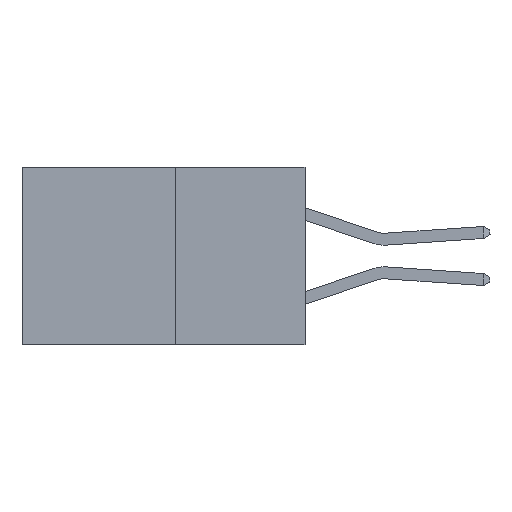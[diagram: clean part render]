
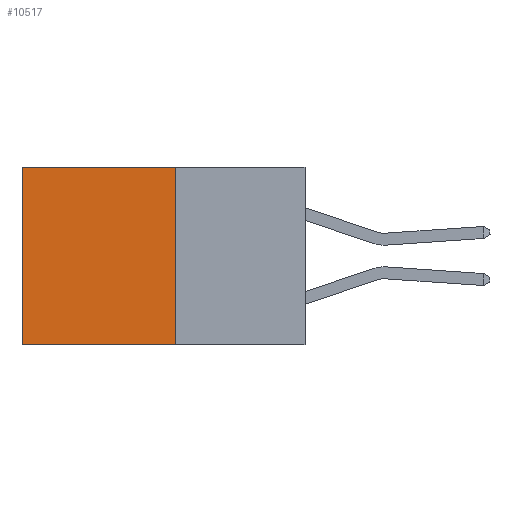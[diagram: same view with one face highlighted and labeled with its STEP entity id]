
A CAD part, left-side view. The second image highlights one B-rep face of the part: STEP entity #10517.
In plain terms, the highlighted planar face has unit normal (-1, 0, 0).
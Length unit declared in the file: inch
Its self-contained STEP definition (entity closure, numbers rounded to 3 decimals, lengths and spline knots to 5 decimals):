
#1689 = VERTEX_POINT ( 'NONE', #20859 ) ;
#1911 = DIRECTION ( 'NONE',  ( 0., 0., -1. ) ) ;
#2279 = ORIENTED_EDGE ( 'NONE', *, *, #21370, .T. ) ;
#2546 = VERTEX_POINT ( 'NONE', #15815 ) ;
#3256 = AXIS2_PLACEMENT_3D ( 'NONE', #24664, #17176, #1911 ) ;
#3782 = VECTOR ( 'NONE', #18553, 39.37008 ) ;
#4202 = VECTOR ( 'NONE', #20544, 39.37008 ) ;
#5334 = EDGE_LOOP ( 'NONE', ( #12758, #12840, #9697, #2279 ) ) ;
#6004 = VECTOR ( 'NONE', #20820, 39.37008 ) ;
#6145 = CARTESIAN_POINT ( 'NONE',  ( 0.277, 0.27, 0. ) ) ;
#6254 = EDGE_CURVE ( 'NONE', #26282, #1689, #18780, .T. ) ;
#9666 = EDGE_CURVE ( 'NONE', #1689, #2546, #29985, .T. ) ;
#9697 = ORIENTED_EDGE ( 'NONE', *, *, #6254, .F. ) ;
#10517 = ADVANCED_FACE ( 'NONE', ( #16028 ), #32265, .F. ) ;
#11269 = CARTESIAN_POINT ( 'NONE',  ( 0.277, 0.27, -0.37 ) ) ;
#11520 = EDGE_CURVE ( 'NONE', #27380, #2546, #28590, .T. ) ;
#12758 = ORIENTED_EDGE ( 'NONE', *, *, #11520, .T. ) ;
#12840 = ORIENTED_EDGE ( 'NONE', *, *, #9666, .F. ) ;
#14352 = VECTOR ( 'NONE', #24694, 39.37008 ) ;
#15496 = CARTESIAN_POINT ( 'NONE',  ( 0.277, 0.27, 0. ) ) ;
#15815 = CARTESIAN_POINT ( 'NONE',  ( 0.277, 0.59, -0.37 ) ) ;
#16012 = CARTESIAN_POINT ( 'NONE',  ( 0.277, 0.27, -0.37 ) ) ;
#16028 = FACE_OUTER_BOUND ( 'NONE', #5334, .T. ) ;
#17101 = CARTESIAN_POINT ( 'NONE',  ( 0.277, 0.59, -0.37 ) ) ;
#17176 = DIRECTION ( 'NONE',  ( 1., 0., 0. ) ) ;
#17772 = LINE ( 'NONE', #15496, #4202 ) ;
#18553 = DIRECTION ( 'NONE',  ( 0., 1., 0. ) ) ;
#18780 = LINE ( 'NONE', #11269, #6004 ) ;
#20544 = DIRECTION ( 'NONE',  ( 0., 1., 0. ) ) ;
#20820 = DIRECTION ( 'NONE',  ( 0., 0., -1. ) ) ;
#20859 = CARTESIAN_POINT ( 'NONE',  ( 0.277, 0.27, -0.37 ) ) ;
#21370 = EDGE_CURVE ( 'NONE', #26282, #27380, #17772, .T. ) ;
#24664 = CARTESIAN_POINT ( 'NONE',  ( 0.277, 0.27, -0.37 ) ) ;
#24694 = DIRECTION ( 'NONE',  ( 0., 0., -1. ) ) ;
#26282 = VERTEX_POINT ( 'NONE', #6145 ) ;
#27380 = VERTEX_POINT ( 'NONE', #31751 ) ;
#28590 = LINE ( 'NONE', #17101, #14352 ) ;
#29985 = LINE ( 'NONE', #16012, #3782 ) ;
#31751 = CARTESIAN_POINT ( 'NONE',  ( 0.277, 0.59, 0. ) ) ;
#32265 = PLANE ( 'NONE',  #3256 ) ;
